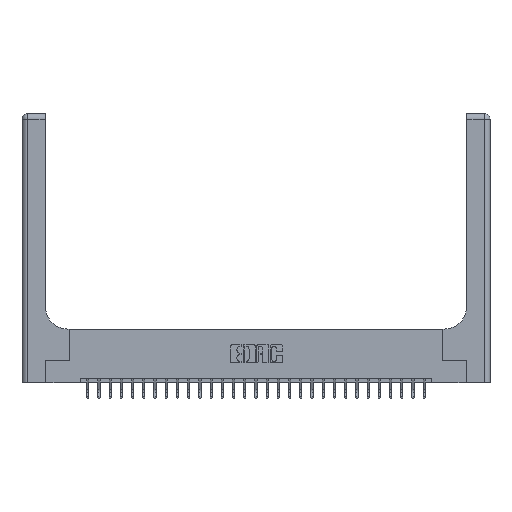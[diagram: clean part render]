
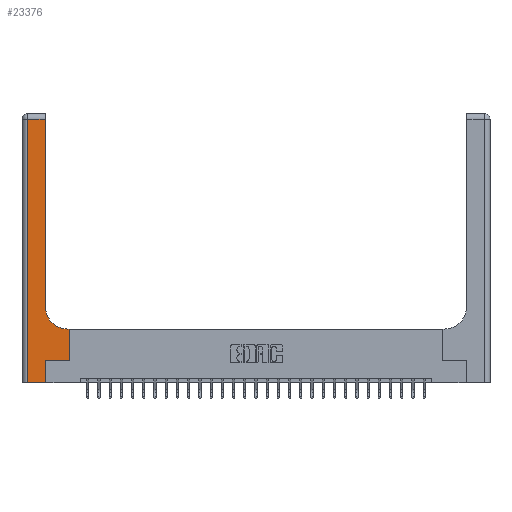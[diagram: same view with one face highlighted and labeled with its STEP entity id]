
A CAD part, top view. The second image highlights one B-rep face of the part: STEP entity #23376.
In plain terms, the highlighted planar face has unit normal (0, 0, 1).
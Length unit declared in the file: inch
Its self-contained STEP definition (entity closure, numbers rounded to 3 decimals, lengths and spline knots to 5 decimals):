
#269 = DIRECTION ( 'NONE',  ( 1., 0., 0. ) ) ;
#289 = VERTEX_POINT ( 'NONE', #26301 ) ;
#744 = LINE ( 'NONE', #12591, #23717 ) ;
#952 = DIRECTION ( 'NONE',  ( -1., 0., 0. ) ) ;
#1211 = ORIENTED_EDGE ( 'NONE', *, *, #17055, .T. ) ;
#1220 = EDGE_CURVE ( 'NONE', #8248, #25673, #24659, .T. ) ;
#1809 = VERTEX_POINT ( 'NONE', #16397 ) ;
#2107 = EDGE_CURVE ( 'NONE', #6900, #16831, #744, .T. ) ;
#2548 = EDGE_CURVE ( 'NONE', #16831, #16955, #19102, .T. ) ;
#2886 = VECTOR ( 'NONE', #13296, 39.37008 ) ;
#3350 = CARTESIAN_POINT ( 'NONE',  ( 0.51, 0.6, 0.37 ) ) ;
#3440 = VECTOR ( 'NONE', #5003, 39.37008 ) ;
#3511 = ORIENTED_EDGE ( 'NONE', *, *, #2107, .T. ) ;
#3617 = DIRECTION ( 'NONE',  ( -1., 0., 0. ) ) ;
#3772 = ORIENTED_EDGE ( 'NONE', *, *, #21749, .T. ) ;
#4155 = EDGE_CURVE ( 'NONE', #24137, #6900, #18684, .T. ) ;
#4936 = PLANE ( 'NONE',  #18824 ) ;
#5003 = DIRECTION ( 'NONE',  ( 0., 1., 0. ) ) ;
#5288 = EDGE_CURVE ( 'NONE', #25673, #1809, #17300, .T. ) ;
#5608 = CARTESIAN_POINT ( 'NONE',  ( 0.265, 0.25, 0.37 ) ) ;
#5873 = CARTESIAN_POINT ( 'NONE',  ( 0.528, 0.25, 0.37 ) ) ;
#6634 = CARTESIAN_POINT ( 'NONE',  ( 0.06, 0., 0.37 ) ) ;
#6900 = VERTEX_POINT ( 'NONE', #25429 ) ;
#7128 = DIRECTION ( 'NONE',  ( 0., 0., -1. ) ) ;
#7306 = DIRECTION ( 'NONE',  ( 0., 1., 0. ) ) ;
#7482 = AXIS2_PLACEMENT_3D ( 'NONE', #10674, #25446, #269 ) ;
#8248 = VERTEX_POINT ( 'NONE', #3350 ) ;
#10516 = CARTESIAN_POINT ( 'NONE',  ( 0.26, 0.85, 0.37 ) ) ;
#10621 = DIRECTION ( 'NONE',  ( 1., 0., 0. ) ) ;
#10648 = ORIENTED_EDGE ( 'NONE', *, *, #1220, .T. ) ;
#10674 = CARTESIAN_POINT ( 'NONE',  ( 0.51, 0.85, 0.37 ) ) ;
#10722 = CARTESIAN_POINT ( 'NONE',  ( 0., 0., 0.37 ) ) ;
#11039 = ORIENTED_EDGE ( 'NONE', *, *, #2548, .T. ) ;
#11628 = ORIENTED_EDGE ( 'NONE', *, *, #4155, .T. ) ;
#12161 = VECTOR ( 'NONE', #13345, 39.37008 ) ;
#12591 = CARTESIAN_POINT ( 'NONE',  ( 0.265, 0., 0.37 ) ) ;
#12609 = LINE ( 'NONE', #13861, #22495 ) ;
#13068 = ORIENTED_EDGE ( 'NONE', *, *, #25376, .T. ) ;
#13296 = DIRECTION ( 'NONE',  ( 0., -1., 0. ) ) ;
#13345 = DIRECTION ( 'NONE',  ( 1., 0., 0. ) ) ;
#13626 = CARTESIAN_POINT ( 'NONE',  ( 0.265, 0.25, 0.37 ) ) ;
#13861 = CARTESIAN_POINT ( 'NONE',  ( 0.528, 0.25, 0.37 ) ) ;
#15528 = CARTESIAN_POINT ( 'NONE',  ( 0., 3., 0.37 ) ) ;
#15546 = VECTOR ( 'NONE', #3617, 39.37008 ) ;
#16370 = VECTOR ( 'NONE', #10621, 39.37008 ) ;
#16397 = CARTESIAN_POINT ( 'NONE',  ( 0.26, 2.94, 0.37 ) ) ;
#16831 = VERTEX_POINT ( 'NONE', #13626 ) ;
#16849 = DIRECTION ( 'NONE',  ( 0., 1., 0. ) ) ;
#16865 = DIRECTION ( 'NONE',  ( -1., 0., 0. ) ) ;
#16955 = VERTEX_POINT ( 'NONE', #5873 ) ;
#17055 = EDGE_CURVE ( 'NONE', #289, #24137, #25902, .T. ) ;
#17139 = CARTESIAN_POINT ( 'NONE',  ( 0.26, 0.6, 0.37 ) ) ;
#17300 = LINE ( 'NONE', #26230, #3440 ) ;
#18031 = FACE_OUTER_BOUND ( 'NONE', #22202, .T. ) ;
#18684 = LINE ( 'NONE', #10722, #16370 ) ;
#18719 = CARTESIAN_POINT ( 'NONE',  ( 0.528, 0.6, 0.37 ) ) ;
#18824 = AXIS2_PLACEMENT_3D ( 'NONE', #15528, #7128, #952 ) ;
#19102 = LINE ( 'NONE', #5608, #12161 ) ;
#20765 = VERTEX_POINT ( 'NONE', #18719 ) ;
#20977 = ORIENTED_EDGE ( 'NONE', *, *, #24586, .T. ) ;
#21594 = LINE ( 'NONE', #17139, #25798 ) ;
#21749 = EDGE_CURVE ( 'NONE', #1809, #289, #22463, .T. ) ;
#22160 = CARTESIAN_POINT ( 'NONE',  ( 0.06, 3., 0.37 ) ) ;
#22202 = EDGE_LOOP ( 'NONE', ( #25100, #3772, #1211, #11628, #3511, #11039, #13068, #20977, #10648 ) ) ;
#22463 = LINE ( 'NONE', #26426, #15546 ) ;
#22495 = VECTOR ( 'NONE', #7306, 39.37008 ) ;
#23376 = ADVANCED_FACE ( 'NONE', ( #18031 ), #4936, .F. ) ;
#23717 = VECTOR ( 'NONE', #16849, 39.37008 ) ;
#24137 = VERTEX_POINT ( 'NONE', #6634 ) ;
#24586 = EDGE_CURVE ( 'NONE', #20765, #8248, #21594, .T. ) ;
#24659 = CIRCLE ( 'NONE', #7482, 0.25 ) ;
#25100 = ORIENTED_EDGE ( 'NONE', *, *, #5288, .T. ) ;
#25376 = EDGE_CURVE ( 'NONE', #16955, #20765, #12609, .T. ) ;
#25429 = CARTESIAN_POINT ( 'NONE',  ( 0.265, 0., 0.37 ) ) ;
#25446 = DIRECTION ( 'NONE',  ( 0., 0., -1. ) ) ;
#25673 = VERTEX_POINT ( 'NONE', #10516 ) ;
#25798 = VECTOR ( 'NONE', #16865, 39.37008 ) ;
#25902 = LINE ( 'NONE', #22160, #2886 ) ;
#26230 = CARTESIAN_POINT ( 'NONE',  ( 0.26, 3., 0.37 ) ) ;
#26301 = CARTESIAN_POINT ( 'NONE',  ( 0.06, 2.94, 0.37 ) ) ;
#26426 = CARTESIAN_POINT ( 'NONE',  ( 0., 2.94, 0.37 ) ) ;
